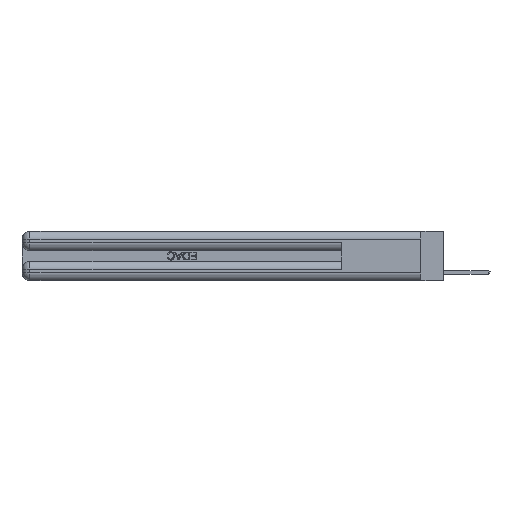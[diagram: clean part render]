
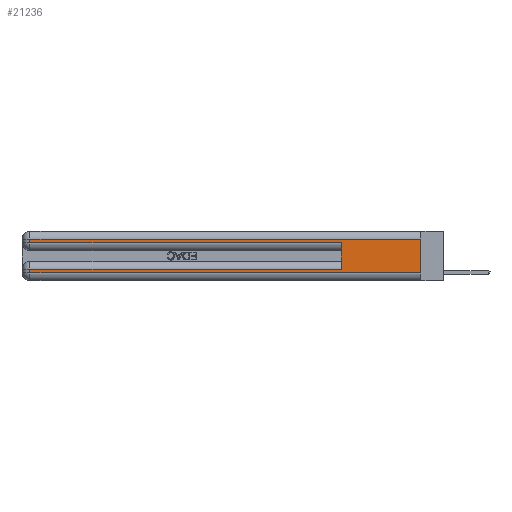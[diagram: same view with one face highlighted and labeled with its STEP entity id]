
A CAD part, left-side view. The second image highlights one B-rep face of the part: STEP entity #21236.
In plain terms, the highlighted planar face has unit normal (-1, 0, 0).
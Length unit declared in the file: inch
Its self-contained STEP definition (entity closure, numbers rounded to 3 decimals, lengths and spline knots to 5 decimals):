
#743 = VERTEX_POINT ( 'NONE', #21997 ) ;
#907 = VECTOR ( 'NONE', #16065, 39.37008 ) ;
#1636 = EDGE_CURVE ( 'NONE', #23505, #19611, #22867, .T. ) ;
#2071 = EDGE_CURVE ( 'NONE', #21947, #743, #17377, .T. ) ;
#2150 = PLANE ( 'NONE',  #13095 ) ;
#2707 = EDGE_CURVE ( 'NONE', #14862, #24313, #26708, .T. ) ;
#3201 = CARTESIAN_POINT ( 'NONE',  ( 0., 2.94, 0.085 ) ) ;
#3224 = VECTOR ( 'NONE', #25124, 39.37008 ) ;
#3528 = CARTESIAN_POINT ( 'NONE',  ( 0., 2.94, 0.06 ) ) ;
#3616 = CARTESIAN_POINT ( 'NONE',  ( 0., 2.94, 0.37 ) ) ;
#4539 = ORIENTED_EDGE ( 'NONE', *, *, #13649, .T. ) ;
#4869 = ORIENTED_EDGE ( 'NONE', *, *, #19452, .F. ) ;
#5088 = LINE ( 'NONE', #6735, #7840 ) ;
#6735 = CARTESIAN_POINT ( 'NONE',  ( 0., 0., 0.31 ) ) ;
#7640 = LINE ( 'NONE', #20047, #17445 ) ;
#7742 = CARTESIAN_POINT ( 'NONE',  ( 0., 2.94, 0.37 ) ) ;
#7840 = VECTOR ( 'NONE', #11227, 39.37008 ) ;
#8400 = CARTESIAN_POINT ( 'NONE',  ( 0., 0., 0.285 ) ) ;
#8687 = CARTESIAN_POINT ( 'NONE',  ( 0., 0., 0.37 ) ) ;
#8820 = LINE ( 'NONE', #14694, #22744 ) ;
#11158 = VECTOR ( 'NONE', #12766, 39.37008 ) ;
#11227 = DIRECTION ( 'NONE',  ( 0., 1., 0. ) ) ;
#11334 = ORIENTED_EDGE ( 'NONE', *, *, #2707, .T. ) ;
#11823 = EDGE_CURVE ( 'NONE', #24313, #743, #14403, .T. ) ;
#12135 = CARTESIAN_POINT ( 'NONE',  ( 0., 2.94, 0.31 ) ) ;
#12766 = DIRECTION ( 'NONE',  ( 0., -1., 0. ) ) ;
#12833 = CARTESIAN_POINT ( 'NONE',  ( 0., 0., 0.37 ) ) ;
#13095 = AXIS2_PLACEMENT_3D ( 'NONE', #8687, #19072, #22645 ) ;
#13452 = CARTESIAN_POINT ( 'NONE',  ( 0., 2.94, 0.285 ) ) ;
#13649 = EDGE_CURVE ( 'NONE', #20027, #14862, #5088, .T. ) ;
#14307 = FACE_OUTER_BOUND ( 'NONE', #22504, .T. ) ;
#14403 = LINE ( 'NONE', #8400, #11158 ) ;
#14617 = LINE ( 'NONE', #12833, #3224 ) ;
#14694 = CARTESIAN_POINT ( 'NONE',  ( 0., 0., 0.085 ) ) ;
#14862 = VERTEX_POINT ( 'NONE', #12135 ) ;
#15236 = ORIENTED_EDGE ( 'NONE', *, *, #21919, .T. ) ;
#15768 = CARTESIAN_POINT ( 'NONE',  ( 0., 0.6, 0.085 ) ) ;
#16065 = DIRECTION ( 'NONE',  ( 0., 0., -1. ) ) ;
#16252 = ORIENTED_EDGE ( 'NONE', *, *, #2071, .F. ) ;
#16771 = ORIENTED_EDGE ( 'NONE', *, *, #1636, .T. ) ;
#17112 = CARTESIAN_POINT ( 'NONE',  ( 0., 0.6, 0.145 ) ) ;
#17377 = LINE ( 'NONE', #17112, #17956 ) ;
#17445 = VECTOR ( 'NONE', #24422, 39.37008 ) ;
#17661 = DIRECTION ( 'NONE',  ( 0., 0., 1. ) ) ;
#17956 = VECTOR ( 'NONE', #17661, 39.37008 ) ;
#19072 = DIRECTION ( 'NONE',  ( 1., 0., 0. ) ) ;
#19452 = EDGE_CURVE ( 'NONE', #20027, #19773, #14617, .T. ) ;
#19611 = VERTEX_POINT ( 'NONE', #3528 ) ;
#19773 = VERTEX_POINT ( 'NONE', #20732 ) ;
#20027 = VERTEX_POINT ( 'NONE', #26543 ) ;
#20047 = CARTESIAN_POINT ( 'NONE',  ( 0., 0., 0.06 ) ) ;
#20393 = DIRECTION ( 'NONE',  ( 0., 0., -1. ) ) ;
#20732 = CARTESIAN_POINT ( 'NONE',  ( 0., 0., 0.06 ) ) ;
#20957 = EDGE_CURVE ( 'NONE', #19611, #19773, #7640, .T. ) ;
#21236 = ADVANCED_FACE ( 'NONE', ( #14307 ), #2150, .F. ) ;
#21901 = VECTOR ( 'NONE', #20393, 39.37008 ) ;
#21919 = EDGE_CURVE ( 'NONE', #21947, #23505, #8820, .T. ) ;
#21947 = VERTEX_POINT ( 'NONE', #15768 ) ;
#21997 = CARTESIAN_POINT ( 'NONE',  ( 0., 0.6, 0.285 ) ) ;
#22216 = ORIENTED_EDGE ( 'NONE', *, *, #20957, .T. ) ;
#22504 = EDGE_LOOP ( 'NONE', ( #4869, #4539, #11334, #26654, #16252, #15236, #16771, #22216 ) ) ;
#22645 = DIRECTION ( 'NONE',  ( 0., 0., -1. ) ) ;
#22744 = VECTOR ( 'NONE', #23030, 39.37008 ) ;
#22867 = LINE ( 'NONE', #3616, #21901 ) ;
#23030 = DIRECTION ( 'NONE',  ( 0., 1., 0. ) ) ;
#23505 = VERTEX_POINT ( 'NONE', #3201 ) ;
#24313 = VERTEX_POINT ( 'NONE', #13452 ) ;
#24422 = DIRECTION ( 'NONE',  ( 0., -1., 0. ) ) ;
#25124 = DIRECTION ( 'NONE',  ( 0., 0., -1. ) ) ;
#26543 = CARTESIAN_POINT ( 'NONE',  ( 0., 0., 0.31 ) ) ;
#26654 = ORIENTED_EDGE ( 'NONE', *, *, #11823, .T. ) ;
#26708 = LINE ( 'NONE', #7742, #907 ) ;
